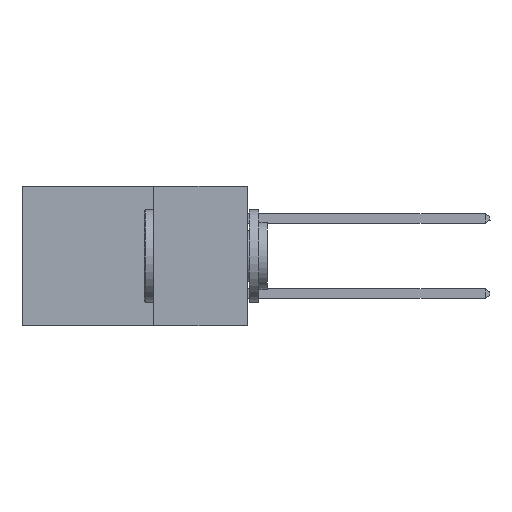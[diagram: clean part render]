
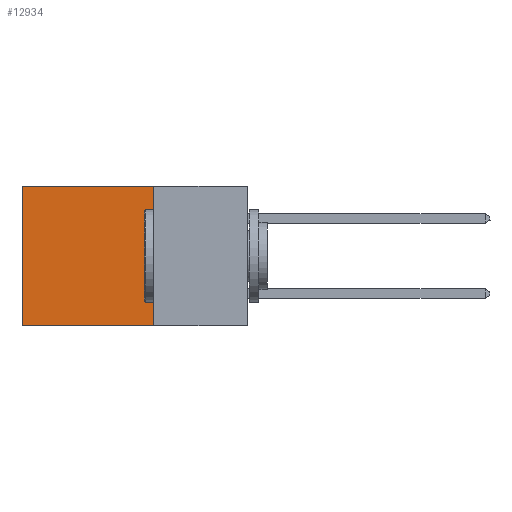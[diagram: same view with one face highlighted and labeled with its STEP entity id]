
A CAD part, left-side view. The second image highlights one B-rep face of the part: STEP entity #12934.
In plain terms, the highlighted planar face has unit normal (-1, 0, 0).
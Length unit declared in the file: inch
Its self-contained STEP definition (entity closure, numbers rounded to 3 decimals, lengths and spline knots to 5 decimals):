
#542 = AXIS2_PLACEMENT_3D ( 'NONE', #22002, #16666, #5836 ) ;
#1722 = EDGE_CURVE ( 'NONE', #23571, #16377, #19601, .T. ) ;
#1865 = LINE ( 'NONE', #16330, #16446 ) ;
#2743 = LINE ( 'NONE', #10520, #11922 ) ;
#3082 = EDGE_CURVE ( 'NONE', #23571, #19883, #1865, .T. ) ;
#3598 = EDGE_LOOP ( 'NONE', ( #12103, #18261, #18637, #14287 ) ) ;
#3971 = PLANE ( 'NONE',  #542 ) ;
#5836 = DIRECTION ( 'NONE',  ( 0., 0., -1. ) ) ;
#6794 = CARTESIAN_POINT ( 'NONE',  ( 0.2615, 0.6, -0.37 ) ) ;
#7385 = EDGE_CURVE ( 'NONE', #19883, #13363, #8101, .T. ) ;
#8076 = CARTESIAN_POINT ( 'NONE',  ( 0.2615, 0.6, 0. ) ) ;
#8101 = LINE ( 'NONE', #6794, #17692 ) ;
#8772 = CARTESIAN_POINT ( 'NONE',  ( 0.2615, 0.6, -0.37 ) ) ;
#9641 = CARTESIAN_POINT ( 'NONE',  ( 0.2615, 0.25, -0.37 ) ) ;
#10444 = DIRECTION ( 'NONE',  ( 0., 0., -1. ) ) ;
#10520 = CARTESIAN_POINT ( 'NONE',  ( 0.2615, 0.25, -0.37 ) ) ;
#11263 = EDGE_CURVE ( 'NONE', #16377, #13363, #2743, .T. ) ;
#11922 = VECTOR ( 'NONE', #19479, 39.37008 ) ;
#12103 = ORIENTED_EDGE ( 'NONE', *, *, #7385, .T. ) ;
#12934 = ADVANCED_FACE ( 'NONE', ( #14068 ), #3971, .F. ) ;
#13363 = VERTEX_POINT ( 'NONE', #8772 ) ;
#14068 = FACE_OUTER_BOUND ( 'NONE', #3598, .T. ) ;
#14287 = ORIENTED_EDGE ( 'NONE', *, *, #3082, .T. ) ;
#15800 = DIRECTION ( 'NONE',  ( 0., 1., 0. ) ) ;
#16074 = CARTESIAN_POINT ( 'NONE',  ( 0.2615, 0.25, -0.37 ) ) ;
#16330 = CARTESIAN_POINT ( 'NONE',  ( 0.2615, 0.25, 0. ) ) ;
#16377 = VERTEX_POINT ( 'NONE', #9641 ) ;
#16446 = VECTOR ( 'NONE', #15800, 39.37008 ) ;
#16666 = DIRECTION ( 'NONE',  ( 1., 0., 0. ) ) ;
#17187 = CARTESIAN_POINT ( 'NONE',  ( 0.2615, 0.25, 0. ) ) ;
#17692 = VECTOR ( 'NONE', #10444, 39.37008 ) ;
#18261 = ORIENTED_EDGE ( 'NONE', *, *, #11263, .F. ) ;
#18637 = ORIENTED_EDGE ( 'NONE', *, *, #1722, .F. ) ;
#19034 = VECTOR ( 'NONE', #22525, 39.37008 ) ;
#19479 = DIRECTION ( 'NONE',  ( 0., 1., 0. ) ) ;
#19601 = LINE ( 'NONE', #16074, #19034 ) ;
#19883 = VERTEX_POINT ( 'NONE', #8076 ) ;
#22002 = CARTESIAN_POINT ( 'NONE',  ( 0.2615, 0.25, -0.37 ) ) ;
#22525 = DIRECTION ( 'NONE',  ( 0., 0., -1. ) ) ;
#23571 = VERTEX_POINT ( 'NONE', #17187 ) ;
